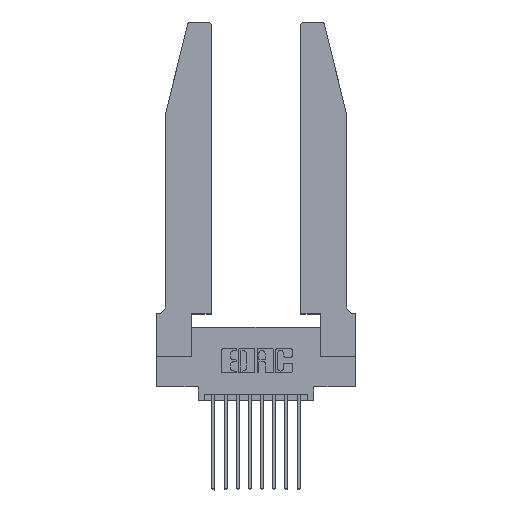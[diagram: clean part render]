
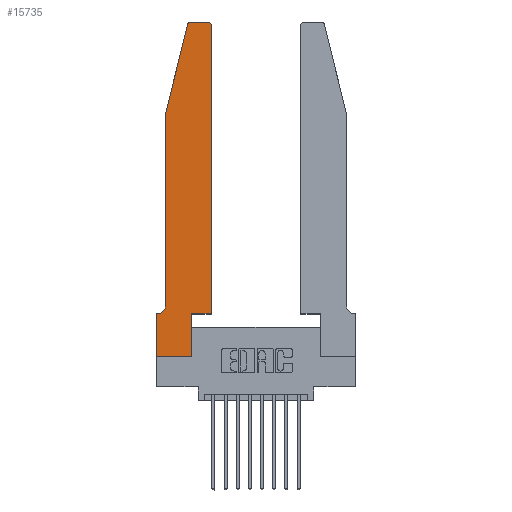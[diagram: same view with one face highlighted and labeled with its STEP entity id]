
A CAD part, top view. The second image highlights one B-rep face of the part: STEP entity #15735.
In plain terms, the highlighted planar face has unit normal (0, 0, 1).
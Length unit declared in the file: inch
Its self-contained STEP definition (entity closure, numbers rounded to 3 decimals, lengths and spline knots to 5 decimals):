
#82 = ORIENTED_EDGE ( 'NONE', *, *, #5974, .T. ) ;
#184 = CIRCLE ( 'NONE', #1762, 0.07 ) ;
#190 = CARTESIAN_POINT ( 'NONE',  ( 0.284, 2.72, 0.37 ) ) ;
#390 = VERTEX_POINT ( 'NONE', #7144 ) ;
#637 = CARTESIAN_POINT ( 'NONE',  ( 0.0755, 2., 0.37 ) ) ;
#788 = VERTEX_POINT ( 'NONE', #5865 ) ;
#811 = DIRECTION ( 'NONE',  ( 0., 0., -1. ) ) ;
#1041 = DIRECTION ( 'NONE',  ( -1., 0., 0. ) ) ;
#1122 = EDGE_CURVE ( 'NONE', #2852, #788, #1458, .T. ) ;
#1208 = ORIENTED_EDGE ( 'NONE', *, *, #6619, .T. ) ;
#1369 = DIRECTION ( 'NONE',  ( 0., 0., 1. ) ) ;
#1458 = LINE ( 'NONE', #11556, #6419 ) ;
#1537 = DIRECTION ( 'NONE',  ( 1., 0., 0. ) ) ;
#1738 = EDGE_CURVE ( 'NONE', #10085, #9564, #2391, .T. ) ;
#1762 = AXIS2_PLACEMENT_3D ( 'NONE', #5358, #811, #13833 ) ;
#1983 = VECTOR ( 'NONE', #14821, 39.37008 ) ;
#2050 = DIRECTION ( 'NONE',  ( 1., 0., 0. ) ) ;
#2291 = CARTESIAN_POINT ( 'NONE',  ( 0.0055, 0.35, 0.37 ) ) ;
#2321 = CARTESIAN_POINT ( 'NONE',  ( 0.2605, 2.75, 0.37 ) ) ;
#2368 = EDGE_CURVE ( 'NONE', #788, #390, #6193, .T. ) ;
#2391 = LINE ( 'NONE', #7929, #5084 ) ;
#2526 = VERTEX_POINT ( 'NONE', #8981 ) ;
#2816 = LINE ( 'NONE', #4318, #7571 ) ;
#2852 = VERTEX_POINT ( 'NONE', #7257 ) ;
#2924 = EDGE_CURVE ( 'NONE', #14094, #2526, #3104, .T. ) ;
#2954 = CARTESIAN_POINT ( 'NONE',  ( 0.25487, 2.72718, 0.37 ) ) ;
#3080 = DIRECTION ( 'NONE',  ( -1., 0., 0. ) ) ;
#3104 = LINE ( 'NONE', #2321, #3904 ) ;
#3177 = DIRECTION ( 'NONE',  ( 0., 0., 1. ) ) ;
#3567 = CIRCLE ( 'NONE', #12333, 0.03 ) ;
#3715 = ORIENTED_EDGE ( 'NONE', *, *, #11586, .T. ) ;
#3845 = ORIENTED_EDGE ( 'NONE', *, *, #11172, .T. ) ;
#3904 = VECTOR ( 'NONE', #1041, 39.37008 ) ;
#3972 = CARTESIAN_POINT ( 'NONE',  ( 0.4205, 2.72, 0.37 ) ) ;
#4318 = CARTESIAN_POINT ( 'NONE',  ( 0.0755, 0.35, 0.37 ) ) ;
#4694 = CARTESIAN_POINT ( 'NONE',  ( 0.2865, 0.35, 0.37 ) ) ;
#4747 = VECTOR ( 'NONE', #15347, 39.37008 ) ;
#5084 = VECTOR ( 'NONE', #9150, 39.37008 ) ;
#5358 = CARTESIAN_POINT ( 'NONE',  ( 0.0055, 0.42, 0.37 ) ) ;
#5812 = VERTEX_POINT ( 'NONE', #4694 ) ;
#5865 = CARTESIAN_POINT ( 'NONE',  ( 0., 0., 0.37 ) ) ;
#5974 = EDGE_CURVE ( 'NONE', #8066, #2852, #2816, .T. ) ;
#6140 = FACE_OUTER_BOUND ( 'NONE', #15770, .T. ) ;
#6157 = VECTOR ( 'NONE', #12895, 39.37008 ) ;
#6175 = CIRCLE ( 'NONE', #13682, 0.03 ) ;
#6193 = LINE ( 'NONE', #6270, #1983 ) ;
#6270 = CARTESIAN_POINT ( 'NONE',  ( 0., 0., 0.37 ) ) ;
#6419 = VECTOR ( 'NONE', #11506, 39.37008 ) ;
#6493 = DIRECTION ( 'NONE',  ( 0., 1., 0. ) ) ;
#6619 = EDGE_CURVE ( 'NONE', #9564, #6625, #11343, .T. ) ;
#6625 = VERTEX_POINT ( 'NONE', #10259 ) ;
#6945 = ORIENTED_EDGE ( 'NONE', *, *, #7691, .T. ) ;
#7144 = CARTESIAN_POINT ( 'NONE',  ( 0.2865, 0., 0.37 ) ) ;
#7257 = CARTESIAN_POINT ( 'NONE',  ( 0., 0.35, 0.37 ) ) ;
#7377 = CARTESIAN_POINT ( 'NONE',  ( 0.4505, 2.72, 0.37 ) ) ;
#7434 = ORIENTED_EDGE ( 'NONE', *, *, #2368, .T. ) ;
#7571 = VECTOR ( 'NONE', #3080, 39.37008 ) ;
#7646 = VERTEX_POINT ( 'NONE', #7377 ) ;
#7691 = EDGE_CURVE ( 'NONE', #2526, #10085, #3567, .T. ) ;
#7816 = DIRECTION ( 'NONE',  ( 0., 1., 0. ) ) ;
#7873 = CARTESIAN_POINT ( 'NONE',  ( 0.2865, 0.35, 0.37 ) ) ;
#7929 = CARTESIAN_POINT ( 'NONE',  ( 0.0755, 2., 0.37 ) ) ;
#8066 = VERTEX_POINT ( 'NONE', #2291 ) ;
#8406 = EDGE_CURVE ( 'NONE', #15678, #7646, #13783, .T. ) ;
#8424 = LINE ( 'NONE', #7873, #13211 ) ;
#8656 = ORIENTED_EDGE ( 'NONE', *, *, #10150, .T. ) ;
#8981 = CARTESIAN_POINT ( 'NONE',  ( 0.284, 2.75, 0.37 ) ) ;
#9150 = DIRECTION ( 'NONE',  ( -0.239, -0.971, 0. ) ) ;
#9152 = CARTESIAN_POINT ( 'NONE',  ( 0.4505, 0.35, 0.37 ) ) ;
#9564 = VERTEX_POINT ( 'NONE', #637 ) ;
#9853 = DIRECTION ( 'NONE',  ( 1., 0., 0. ) ) ;
#10059 = AXIS2_PLACEMENT_3D ( 'NONE', #12855, #3177, #2050 ) ;
#10085 = VERTEX_POINT ( 'NONE', #2954 ) ;
#10150 = EDGE_CURVE ( 'NONE', #390, #5812, #8424, .T. ) ;
#10259 = CARTESIAN_POINT ( 'NONE',  ( 0.0755, 0.42, 0.37 ) ) ;
#10914 = VECTOR ( 'NONE', #6493, 39.37008 ) ;
#11043 = ORIENTED_EDGE ( 'NONE', *, *, #1738, .T. ) ;
#11172 = EDGE_CURVE ( 'NONE', #7646, #14094, #6175, .T. ) ;
#11313 = CARTESIAN_POINT ( 'NONE',  ( 0.4505, 0.35, 0.37 ) ) ;
#11343 = LINE ( 'NONE', #12114, #4747 ) ;
#11457 = CARTESIAN_POINT ( 'NONE',  ( 0.4505, 0.35, 0.37 ) ) ;
#11506 = DIRECTION ( 'NONE',  ( 0., -1., 0. ) ) ;
#11556 = CARTESIAN_POINT ( 'NONE',  ( 0., 0., 0.37 ) ) ;
#11586 = EDGE_CURVE ( 'NONE', #5812, #15678, #13378, .T. ) ;
#11626 = PLANE ( 'NONE',  #10059 ) ;
#12114 = CARTESIAN_POINT ( 'NONE',  ( 0.0755, 2., 0.37 ) ) ;
#12182 = ORIENTED_EDGE ( 'NONE', *, *, #12632, .T. ) ;
#12333 = AXIS2_PLACEMENT_3D ( 'NONE', #190, #1369, #9853 ) ;
#12632 = EDGE_CURVE ( 'NONE', #6625, #8066, #184, .T. ) ;
#12855 = CARTESIAN_POINT ( 'NONE',  ( 0., 0.35, 0.37 ) ) ;
#12895 = DIRECTION ( 'NONE',  ( 1., 0., 0. ) ) ;
#13211 = VECTOR ( 'NONE', #7816, 39.37008 ) ;
#13378 = LINE ( 'NONE', #9152, #6157 ) ;
#13586 = DIRECTION ( 'NONE',  ( 0., 0., 1. ) ) ;
#13682 = AXIS2_PLACEMENT_3D ( 'NONE', #3972, #13586, #1537 ) ;
#13783 = LINE ( 'NONE', #11313, #10914 ) ;
#13833 = DIRECTION ( 'NONE',  ( -1., 0., 0. ) ) ;
#13978 = ORIENTED_EDGE ( 'NONE', *, *, #1122, .T. ) ;
#14094 = VERTEX_POINT ( 'NONE', #14770 ) ;
#14510 = ORIENTED_EDGE ( 'NONE', *, *, #8406, .T. ) ;
#14745 = ORIENTED_EDGE ( 'NONE', *, *, #2924, .T. ) ;
#14770 = CARTESIAN_POINT ( 'NONE',  ( 0.4205, 2.75, 0.37 ) ) ;
#14821 = DIRECTION ( 'NONE',  ( 1., 0., 0. ) ) ;
#15347 = DIRECTION ( 'NONE',  ( 0., -1., 0. ) ) ;
#15678 = VERTEX_POINT ( 'NONE', #11457 ) ;
#15735 = ADVANCED_FACE ( 'NONE', ( #6140 ), #11626, .T. ) ;
#15770 = EDGE_LOOP ( 'NONE', ( #14745, #6945, #11043, #1208, #12182, #82, #13978, #7434, #8656, #3715, #14510, #3845 ) ) ;
